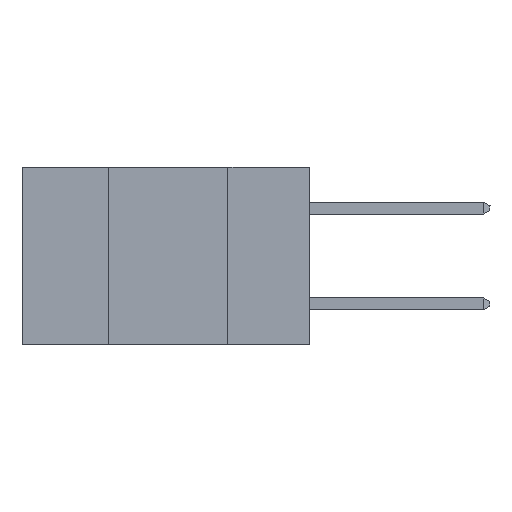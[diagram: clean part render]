
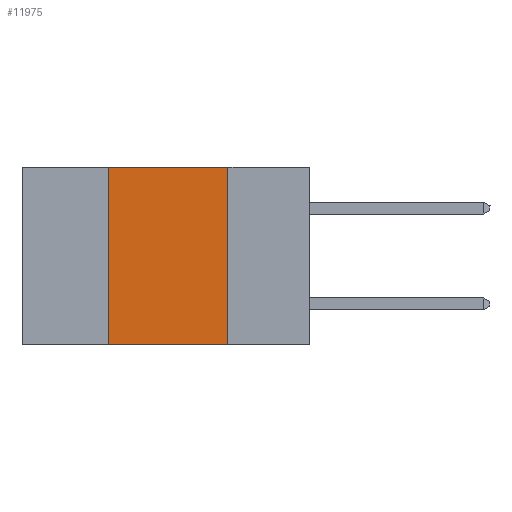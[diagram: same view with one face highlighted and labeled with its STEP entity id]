
A CAD part, left-side view. The second image highlights one B-rep face of the part: STEP entity #11975.
In plain terms, the highlighted planar face has unit normal (-1, 0, 0).
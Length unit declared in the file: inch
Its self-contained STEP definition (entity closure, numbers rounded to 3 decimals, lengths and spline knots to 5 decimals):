
#839 = VERTEX_POINT ( 'NONE', #10219 ) ;
#1551 = CARTESIAN_POINT ( 'NONE',  ( 0., 0.6, 0. ) ) ;
#2181 = ORIENTED_EDGE ( 'NONE', *, *, #31156, .F. ) ;
#5064 = VERTEX_POINT ( 'NONE', #24538 ) ;
#5073 = DIRECTION ( 'NONE',  ( 0., 0., -1. ) ) ;
#5269 = DIRECTION ( 'NONE',  ( 0., -1., 0. ) ) ;
#5985 = ORIENTED_EDGE ( 'NONE', *, *, #27935, .F. ) ;
#6643 = DIRECTION ( 'NONE',  ( 0., 0., 1. ) ) ;
#6762 = LINE ( 'NONE', #10330, #34765 ) ;
#8388 = AXIS2_PLACEMENT_3D ( 'NONE', #45077, #26985, #5073 ) ;
#9615 = EDGE_CURVE ( 'NONE', #5064, #839, #31418, .T. ) ;
#10080 = EDGE_CURVE ( 'NONE', #42552, #839, #11957, .T. ) ;
#10219 = CARTESIAN_POINT ( 'NONE',  ( 0., 0.17, -0.37 ) ) ;
#10330 = CARTESIAN_POINT ( 'NONE',  ( 0., 0.42, 0. ) ) ;
#11722 = VECTOR ( 'NONE', #5269, 39.37008 ) ;
#11957 = LINE ( 'NONE', #15569, #45122 ) ;
#11975 = ADVANCED_FACE ( 'NONE', ( #19121 ), #23348, .F. ) ;
#15569 = CARTESIAN_POINT ( 'NONE',  ( 0., 0.6, -0.37 ) ) ;
#16879 = CARTESIAN_POINT ( 'NONE',  ( 0., 0.17, 0. ) ) ;
#19121 = FACE_OUTER_BOUND ( 'NONE', #35236, .T. ) ;
#23348 = PLANE ( 'NONE',  #8388 ) ;
#24538 = CARTESIAN_POINT ( 'NONE',  ( 0., 0.17, 0. ) ) ;
#26985 = DIRECTION ( 'NONE',  ( 1., 0., 0. ) ) ;
#27935 = EDGE_CURVE ( 'NONE', #42552, #45059, #6762, .T. ) ;
#29292 = CARTESIAN_POINT ( 'NONE',  ( 0., 0.42, 0. ) ) ;
#30259 = DIRECTION ( 'NONE',  ( 0., -1., 0. ) ) ;
#30283 = VECTOR ( 'NONE', #45954, 39.37008 ) ;
#31156 = EDGE_CURVE ( 'NONE', #45059, #5064, #40781, .T. ) ;
#31418 = LINE ( 'NONE', #16879, #30283 ) ;
#33788 = CARTESIAN_POINT ( 'NONE',  ( 0., 0.42, -0.37 ) ) ;
#34765 = VECTOR ( 'NONE', #6643, 39.37008 ) ;
#35236 = EDGE_LOOP ( 'NONE', ( #44931, #2181, #5985, #38537 ) ) ;
#38537 = ORIENTED_EDGE ( 'NONE', *, *, #10080, .T. ) ;
#40781 = LINE ( 'NONE', #1551, #11722 ) ;
#42552 = VERTEX_POINT ( 'NONE', #33788 ) ;
#44931 = ORIENTED_EDGE ( 'NONE', *, *, #9615, .F. ) ;
#45059 = VERTEX_POINT ( 'NONE', #29292 ) ;
#45077 = CARTESIAN_POINT ( 'NONE',  ( 0., 0.6, 0. ) ) ;
#45122 = VECTOR ( 'NONE', #30259, 39.37008 ) ;
#45954 = DIRECTION ( 'NONE',  ( 0., 0., -1. ) ) ;
